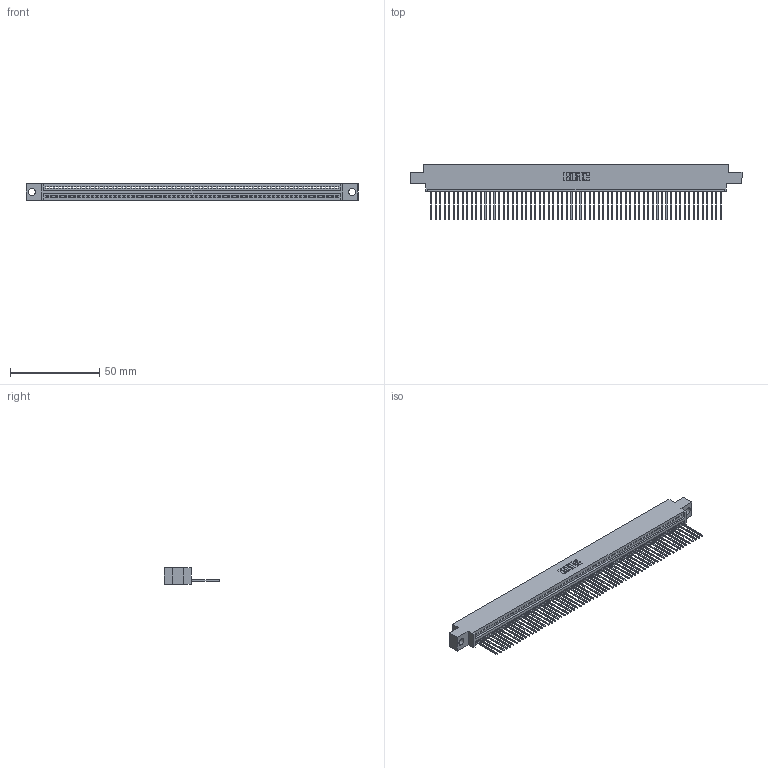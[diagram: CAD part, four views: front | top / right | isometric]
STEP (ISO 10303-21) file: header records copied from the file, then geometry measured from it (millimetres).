
FILE_DESCRIPTION (( 'STEP AP203' ), '1' );
FILE_NAME ('395-065-542-604.STEP', '2021-05-31T22:04:00', ( '' ), ( '' ), 'SwSTEP 2.0', 'SolidWorks 2020', '' );
FILE_SCHEMA (( 'CONFIG_CONTROL_DESIGN' ));
Length unit declared in the file: inch
Products named in the file (3): 395-065-542-604; 345-292-001_345-293-142; 345 Part_0.170 Offset - 0.156 Dia-TI
Assembly tree (66 placements, depth 2):
  395-065-542-604
    345 Part_0.170 Offset - 0.156 Dia-TI
    345-292-001_345-293-142  x65
Bounding box: 186.31 x 31.29 x 9.4 mm (x, y, z)
Volume: 17809.5 mm3; surface area: 24863.4 mm2
Topology: 66 solids, 66 shells, 3914 faces, 11829 edges, 7798 vertices
Faces by surface type: plane 2698, cylinder 1216
Entity records: 46393 total; most frequent: CARTESIAN_POINT 8045, ORIENTED_EDGE 8042, DIRECTION 6991, EDGE_CURVE 4021, VECTOR 3629, LINE 3629, VERTEX_POINT 2678, AXIS2_PLACEMENT_3D 1681
